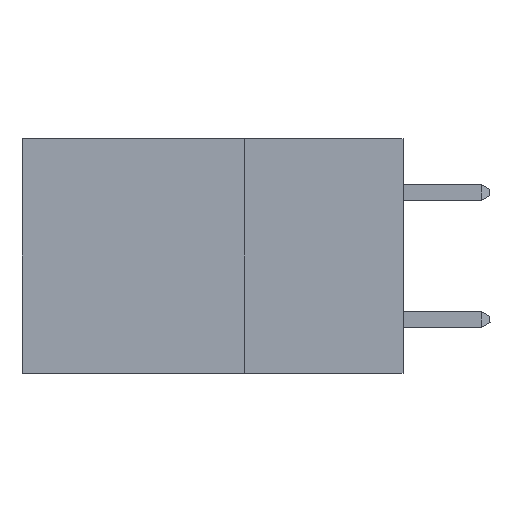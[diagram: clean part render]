
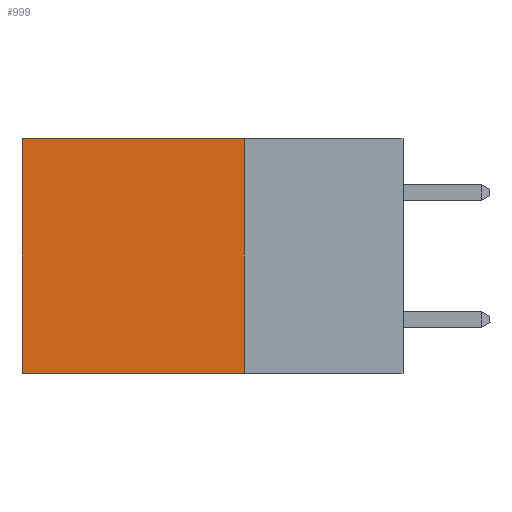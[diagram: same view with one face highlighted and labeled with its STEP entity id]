
A CAD part, left-side view. The second image highlights one B-rep face of the part: STEP entity #999.
In plain terms, the highlighted planar face has unit normal (-1, 0, 0).
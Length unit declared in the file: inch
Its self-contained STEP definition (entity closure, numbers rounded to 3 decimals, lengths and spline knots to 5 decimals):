
#999 = ADVANCED_FACE ( 'NONE', ( #18677 ), #14482, .F. ) ;
#1069 = LINE ( 'NONE', #22659, #3510 ) ;
#1827 = CARTESIAN_POINT ( 'NONE',  ( 0.2875, 0.25, 0. ) ) ;
#2823 = DIRECTION ( 'NONE',  ( 0., 0., -1. ) ) ;
#3007 = EDGE_CURVE ( 'NONE', #16989, #7933, #20107, .T. ) ;
#3147 = LINE ( 'NONE', #15985, #3438 ) ;
#3438 = VECTOR ( 'NONE', #17931, 39.37008 ) ;
#3510 = VECTOR ( 'NONE', #6997, 39.37008 ) ;
#3657 = ORIENTED_EDGE ( 'NONE', *, *, #5299, .T. ) ;
#4440 = ORIENTED_EDGE ( 'NONE', *, *, #22369, .T. ) ;
#5059 = EDGE_CURVE ( 'NONE', #7933, #17654, #3147, .T. ) ;
#5299 = EDGE_CURVE ( 'NONE', #9378, #17654, #20759, .T. ) ;
#6997 = DIRECTION ( 'NONE',  ( 0., 1., 0. ) ) ;
#7765 = ORIENTED_EDGE ( 'NONE', *, *, #5059, .F. ) ;
#7933 = VERTEX_POINT ( 'NONE', #11785 ) ;
#9378 = VERTEX_POINT ( 'NONE', #21956 ) ;
#9412 = CARTESIAN_POINT ( 'NONE',  ( 0.2875, 0.6, 0. ) ) ;
#9509 = ORIENTED_EDGE ( 'NONE', *, *, #3007, .F. ) ;
#11785 = CARTESIAN_POINT ( 'NONE',  ( 0.2875, 0.25, -0.37 ) ) ;
#11883 = DIRECTION ( 'NONE',  ( 0., 0., -1. ) ) ;
#12160 = AXIS2_PLACEMENT_3D ( 'NONE', #12776, #20331, #2823 ) ;
#12776 = CARTESIAN_POINT ( 'NONE',  ( 0.2875, 0.25, 0. ) ) ;
#13477 = VECTOR ( 'NONE', #11883, 39.37008 ) ;
#14482 = PLANE ( 'NONE',  #12160 ) ;
#14648 = VECTOR ( 'NONE', #15284, 39.37008 ) ;
#15284 = DIRECTION ( 'NONE',  ( 0., 0., -1. ) ) ;
#15985 = CARTESIAN_POINT ( 'NONE',  ( 0.2875, 0.25, -0.37 ) ) ;
#16989 = VERTEX_POINT ( 'NONE', #17266 ) ;
#17121 = CARTESIAN_POINT ( 'NONE',  ( 0.2875, 0.6, -0.37 ) ) ;
#17266 = CARTESIAN_POINT ( 'NONE',  ( 0.2875, 0.25, 0. ) ) ;
#17654 = VERTEX_POINT ( 'NONE', #17121 ) ;
#17931 = DIRECTION ( 'NONE',  ( 0., 1., 0. ) ) ;
#18677 = FACE_OUTER_BOUND ( 'NONE', #20763, .T. ) ;
#20107 = LINE ( 'NONE', #1827, #14648 ) ;
#20331 = DIRECTION ( 'NONE',  ( 1., 0., 0. ) ) ;
#20759 = LINE ( 'NONE', #9412, #13477 ) ;
#20763 = EDGE_LOOP ( 'NONE', ( #3657, #7765, #9509, #4440 ) ) ;
#21956 = CARTESIAN_POINT ( 'NONE',  ( 0.2875, 0.6, 0. ) ) ;
#22369 = EDGE_CURVE ( 'NONE', #16989, #9378, #1069, .T. ) ;
#22659 = CARTESIAN_POINT ( 'NONE',  ( 0.2875, 0.25, 0. ) ) ;
